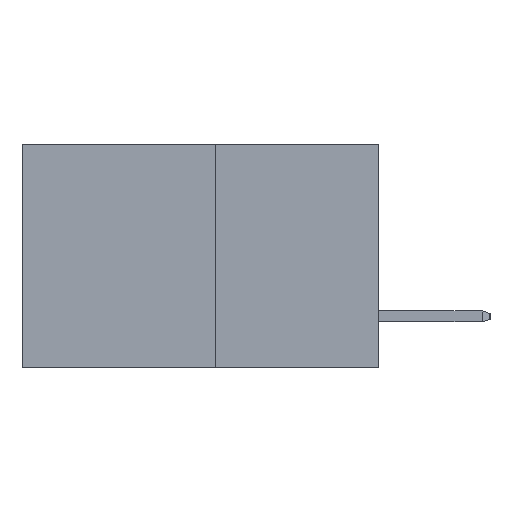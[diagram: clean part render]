
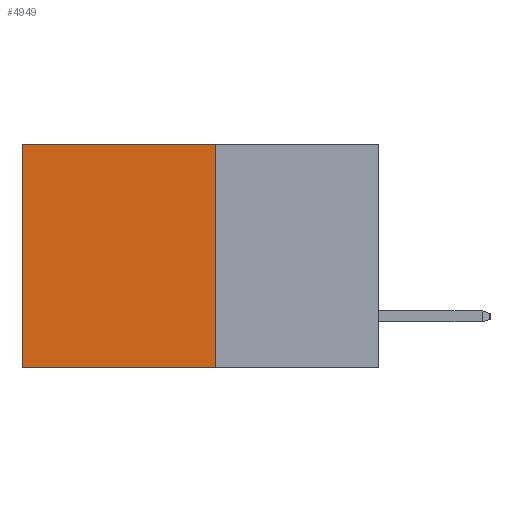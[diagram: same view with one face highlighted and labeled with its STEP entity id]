
A CAD part, left-side view. The second image highlights one B-rep face of the part: STEP entity #4949.
In plain terms, the highlighted planar face has unit normal (-1, 0, 0).
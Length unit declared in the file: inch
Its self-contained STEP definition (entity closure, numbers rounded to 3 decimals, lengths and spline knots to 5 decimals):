
#162 = EDGE_LOOP ( 'NONE', ( #13835, #10221, #22387, #7465 ) ) ;
#783 = DIRECTION ( 'NONE',  ( 0., 0., -1. ) ) ;
#1169 = LINE ( 'NONE', #25721, #10869 ) ;
#3936 = EDGE_CURVE ( 'NONE', #25246, #22349, #28271, .T. ) ;
#4180 = VECTOR ( 'NONE', #4513, 39.37008 ) ;
#4513 = DIRECTION ( 'NONE',  ( 0., 0., -1. ) ) ;
#4949 = ADVANCED_FACE ( 'NONE', ( #23438 ), #11860, .F. ) ;
#5461 = VECTOR ( 'NONE', #19535, 39.37008 ) ;
#5583 = CARTESIAN_POINT ( 'NONE',  ( 0.277, 0.59, -0.37 ) ) ;
#7465 = ORIENTED_EDGE ( 'NONE', *, *, #16280, .T. ) ;
#7703 = LINE ( 'NONE', #23260, #18851 ) ;
#8204 = CARTESIAN_POINT ( 'NONE',  ( 0.277, 0.27, 0. ) ) ;
#8275 = EDGE_CURVE ( 'NONE', #17093, #16663, #21898, .T. ) ;
#8975 = CARTESIAN_POINT ( 'NONE',  ( 0.277, 0.27, -0.37 ) ) ;
#10221 = ORIENTED_EDGE ( 'NONE', *, *, #15016, .F. ) ;
#10869 = VECTOR ( 'NONE', #17007, 39.37008 ) ;
#11860 = PLANE ( 'NONE',  #24302 ) ;
#12605 = CARTESIAN_POINT ( 'NONE',  ( 0.277, 0.59, 0. ) ) ;
#13835 = ORIENTED_EDGE ( 'NONE', *, *, #3936, .T. ) ;
#14077 = DIRECTION ( 'NONE',  ( 1., 0., 0. ) ) ;
#15016 = EDGE_CURVE ( 'NONE', #16663, #22349, #1169, .T. ) ;
#15025 = CARTESIAN_POINT ( 'NONE',  ( 0.277, 0.59, -0.37 ) ) ;
#15566 = CARTESIAN_POINT ( 'NONE',  ( 0.277, 0.27, -0.37 ) ) ;
#16280 = EDGE_CURVE ( 'NONE', #17093, #25246, #7703, .T. ) ;
#16663 = VERTEX_POINT ( 'NONE', #8975 ) ;
#17007 = DIRECTION ( 'NONE',  ( 0., 1., 0. ) ) ;
#17093 = VERTEX_POINT ( 'NONE', #8204 ) ;
#18851 = VECTOR ( 'NONE', #25475, 39.37008 ) ;
#19535 = DIRECTION ( 'NONE',  ( 0., 0., -1. ) ) ;
#21898 = LINE ( 'NONE', #15566, #4180 ) ;
#22349 = VERTEX_POINT ( 'NONE', #5583 ) ;
#22387 = ORIENTED_EDGE ( 'NONE', *, *, #8275, .F. ) ;
#23260 = CARTESIAN_POINT ( 'NONE',  ( 0.277, 0.27, 0. ) ) ;
#23438 = FACE_OUTER_BOUND ( 'NONE', #162, .T. ) ;
#24302 = AXIS2_PLACEMENT_3D ( 'NONE', #25162, #14077, #783 ) ;
#25162 = CARTESIAN_POINT ( 'NONE',  ( 0.277, 0.27, -0.37 ) ) ;
#25246 = VERTEX_POINT ( 'NONE', #12605 ) ;
#25475 = DIRECTION ( 'NONE',  ( 0., 1., 0. ) ) ;
#25721 = CARTESIAN_POINT ( 'NONE',  ( 0.277, 0.27, -0.37 ) ) ;
#28271 = LINE ( 'NONE', #15025, #5461 ) ;
